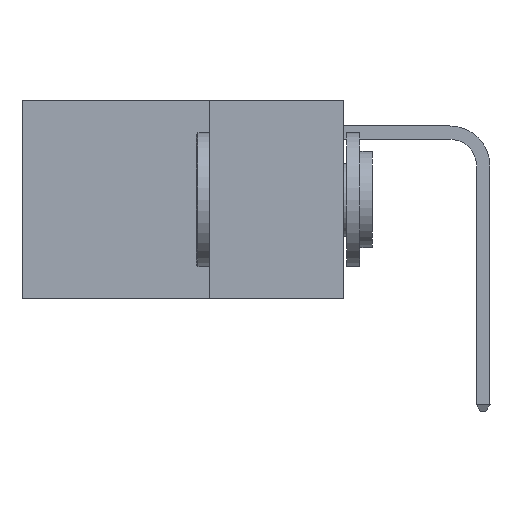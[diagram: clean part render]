
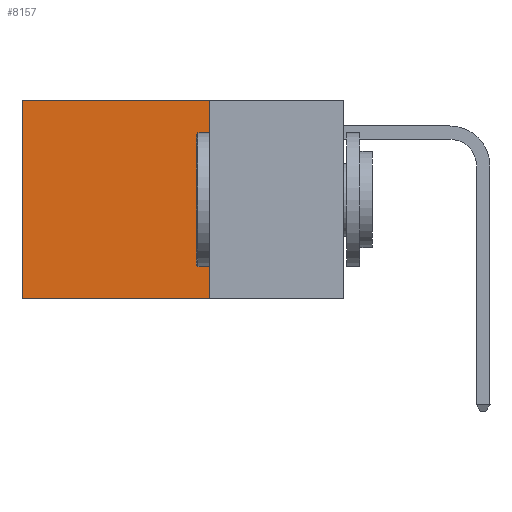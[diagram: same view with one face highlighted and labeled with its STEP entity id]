
A CAD part, left-side view. The second image highlights one B-rep face of the part: STEP entity #8157.
In plain terms, the highlighted planar face has unit normal (-1, 0, 0).
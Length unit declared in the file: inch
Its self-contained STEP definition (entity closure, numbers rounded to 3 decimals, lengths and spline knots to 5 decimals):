
#1906 = LINE ( 'NONE', #13534, #8342 ) ;
#2240 = LINE ( 'NONE', #11181, #5272 ) ;
#2787 = VERTEX_POINT ( 'NONE', #4290 ) ;
#3098 = PLANE ( 'NONE',  #12502 ) ;
#3420 = EDGE_CURVE ( 'NONE', #15863, #2787, #1906, .T. ) ;
#3462 = CARTESIAN_POINT ( 'NONE',  ( 0.2625, 0.25, 0. ) ) ;
#3801 = EDGE_CURVE ( 'NONE', #10920, #2787, #13081, .T. ) ;
#4290 = CARTESIAN_POINT ( 'NONE',  ( 0.2625, 0.6, -0.37 ) ) ;
#4401 = CARTESIAN_POINT ( 'NONE',  ( 0.2625, 0.25, 0. ) ) ;
#5192 = VERTEX_POINT ( 'NONE', #10036 ) ;
#5272 = VECTOR ( 'NONE', #12583, 39.37008 ) ;
#5712 = DIRECTION ( 'NONE',  ( 0., 0., -1. ) ) ;
#6112 = VECTOR ( 'NONE', #14697, 39.37008 ) ;
#6261 = FACE_OUTER_BOUND ( 'NONE', #15560, .T. ) ;
#7876 = CARTESIAN_POINT ( 'NONE',  ( 0.2625, 0.6, 0. ) ) ;
#8157 = ADVANCED_FACE ( 'NONE', ( #6261 ), #3098, .F. ) ;
#8342 = VECTOR ( 'NONE', #13642, 39.37008 ) ;
#9202 = CARTESIAN_POINT ( 'NONE',  ( 0.2625, 0.25, -0.37 ) ) ;
#9292 = LINE ( 'NONE', #3462, #12824 ) ;
#9637 = ORIENTED_EDGE ( 'NONE', *, *, #3801, .F. ) ;
#10036 = CARTESIAN_POINT ( 'NONE',  ( 0.2625, 0.25, 0. ) ) ;
#10920 = VERTEX_POINT ( 'NONE', #9202 ) ;
#11181 = CARTESIAN_POINT ( 'NONE',  ( 0.2625, 0.25, 0. ) ) ;
#11256 = DIRECTION ( 'NONE',  ( 0., 1., 0. ) ) ;
#11822 = ORIENTED_EDGE ( 'NONE', *, *, #14932, .F. ) ;
#12201 = ORIENTED_EDGE ( 'NONE', *, *, #3420, .T. ) ;
#12502 = AXIS2_PLACEMENT_3D ( 'NONE', #4401, #13519, #5712 ) ;
#12583 = DIRECTION ( 'NONE',  ( 0., 0., -1. ) ) ;
#12824 = VECTOR ( 'NONE', #11256, 39.37008 ) ;
#13046 = ORIENTED_EDGE ( 'NONE', *, *, #14429, .T. ) ;
#13081 = LINE ( 'NONE', #14740, #6112 ) ;
#13519 = DIRECTION ( 'NONE',  ( 1., 0., 0. ) ) ;
#13534 = CARTESIAN_POINT ( 'NONE',  ( 0.2625, 0.6, 0. ) ) ;
#13642 = DIRECTION ( 'NONE',  ( 0., 0., -1. ) ) ;
#14429 = EDGE_CURVE ( 'NONE', #5192, #15863, #9292, .T. ) ;
#14697 = DIRECTION ( 'NONE',  ( 0., 1., 0. ) ) ;
#14740 = CARTESIAN_POINT ( 'NONE',  ( 0.2625, 0.25, -0.37 ) ) ;
#14932 = EDGE_CURVE ( 'NONE', #5192, #10920, #2240, .T. ) ;
#15560 = EDGE_LOOP ( 'NONE', ( #12201, #9637, #11822, #13046 ) ) ;
#15863 = VERTEX_POINT ( 'NONE', #7876 ) ;
